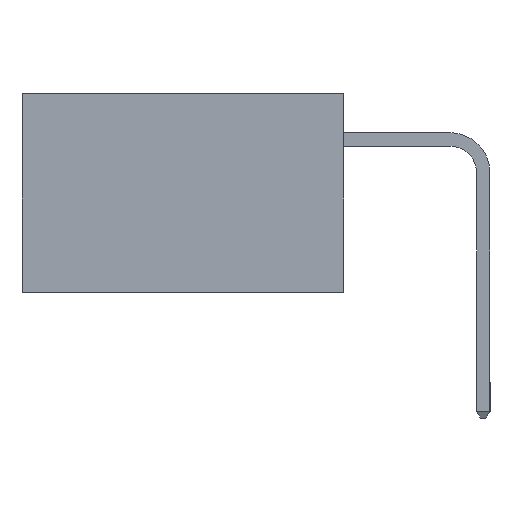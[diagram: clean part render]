
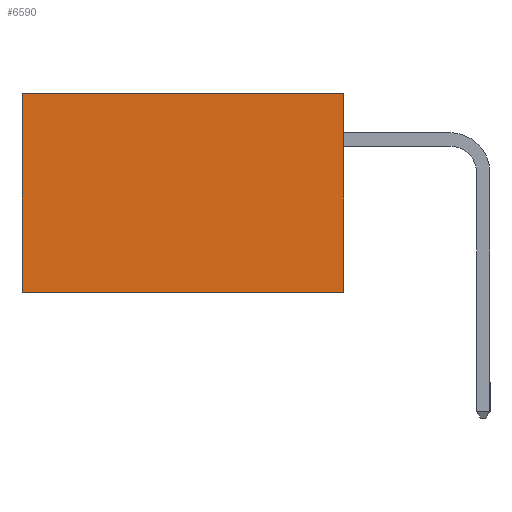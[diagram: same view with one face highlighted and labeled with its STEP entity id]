
A CAD part, left-side view. The second image highlights one B-rep face of the part: STEP entity #6590.
In plain terms, the highlighted planar face has unit normal (-1, 0, 0).
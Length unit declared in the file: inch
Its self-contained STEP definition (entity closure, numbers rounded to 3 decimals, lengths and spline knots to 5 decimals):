
#142 = CARTESIAN_POINT ( 'NONE',  ( 0.2615, 0.6, -0.37 ) ) ;
#184 = LINE ( 'NONE', #529, #18989 ) ;
#529 = CARTESIAN_POINT ( 'NONE',  ( 0.2615, 0., 0. ) ) ;
#1098 = VECTOR ( 'NONE', #2996, 39.37008 ) ;
#1259 = LINE ( 'NONE', #15757, #1098 ) ;
#1563 = VECTOR ( 'NONE', #20880, 39.37008 ) ;
#2996 = DIRECTION ( 'NONE',  ( 0., 1., 0. ) ) ;
#3347 = AXIS2_PLACEMENT_3D ( 'NONE', #12802, #4256, #11358 ) ;
#4256 = DIRECTION ( 'NONE',  ( 1., 0., 0. ) ) ;
#4358 = FACE_OUTER_BOUND ( 'NONE', #18199, .T. ) ;
#5499 = VERTEX_POINT ( 'NONE', #142 ) ;
#6139 = DIRECTION ( 'NONE',  ( 0., 0., -1. ) ) ;
#6453 = EDGE_CURVE ( 'NONE', #21141, #5499, #1259, .T. ) ;
#6590 = ADVANCED_FACE ( 'NONE', ( #4358 ), #18499, .F. ) ;
#6604 = CARTESIAN_POINT ( 'NONE',  ( 0.2615, 0., -0.37 ) ) ;
#8746 = CARTESIAN_POINT ( 'NONE',  ( 0.2615, 0.6, 0. ) ) ;
#10316 = VERTEX_POINT ( 'NONE', #13784 ) ;
#11358 = DIRECTION ( 'NONE',  ( 0., 0., -1. ) ) ;
#12646 = ORIENTED_EDGE ( 'NONE', *, *, #18617, .T. ) ;
#12802 = CARTESIAN_POINT ( 'NONE',  ( 0.2615, 0., -0.37 ) ) ;
#13471 = EDGE_CURVE ( 'NONE', #10316, #21141, #13735, .T. ) ;
#13735 = LINE ( 'NONE', #22861, #1563 ) ;
#13784 = CARTESIAN_POINT ( 'NONE',  ( 0.2615, 0., 0. ) ) ;
#14427 = DIRECTION ( 'NONE',  ( 0., 1., 0. ) ) ;
#15472 = VERTEX_POINT ( 'NONE', #8746 ) ;
#15757 = CARTESIAN_POINT ( 'NONE',  ( 0.2615, 0., -0.37 ) ) ;
#16007 = VECTOR ( 'NONE', #6139, 39.37008 ) ;
#16925 = ORIENTED_EDGE ( 'NONE', *, *, #13471, .F. ) ;
#18199 = EDGE_LOOP ( 'NONE', ( #12646, #22149, #16925, #22772 ) ) ;
#18499 = PLANE ( 'NONE',  #3347 ) ;
#18617 = EDGE_CURVE ( 'NONE', #15472, #5499, #22511, .T. ) ;
#18980 = CARTESIAN_POINT ( 'NONE',  ( 0.2615, 0.6, -0.37 ) ) ;
#18989 = VECTOR ( 'NONE', #14427, 39.37008 ) ;
#18995 = EDGE_CURVE ( 'NONE', #10316, #15472, #184, .T. ) ;
#20880 = DIRECTION ( 'NONE',  ( 0., 0., -1. ) ) ;
#21141 = VERTEX_POINT ( 'NONE', #6604 ) ;
#22149 = ORIENTED_EDGE ( 'NONE', *, *, #6453, .F. ) ;
#22511 = LINE ( 'NONE', #18980, #16007 ) ;
#22772 = ORIENTED_EDGE ( 'NONE', *, *, #18995, .T. ) ;
#22861 = CARTESIAN_POINT ( 'NONE',  ( 0.2615, 0., -0.37 ) ) ;
